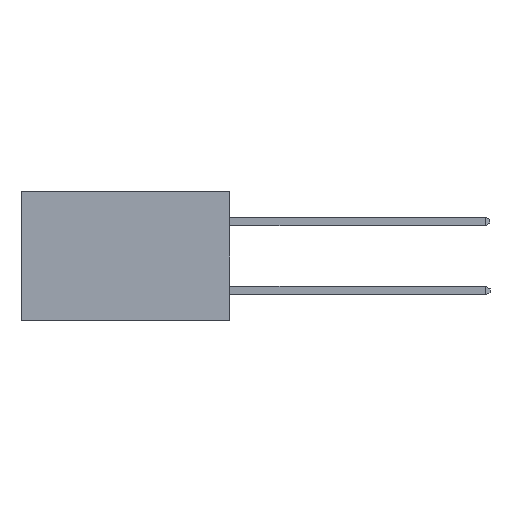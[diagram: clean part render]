
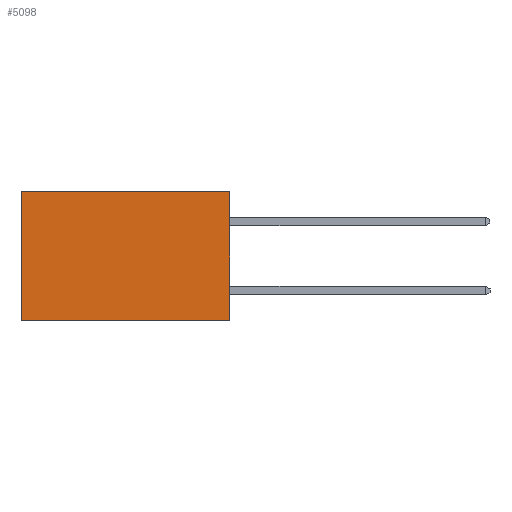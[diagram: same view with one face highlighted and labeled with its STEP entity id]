
A CAD part, left-side view. The second image highlights one B-rep face of the part: STEP entity #5098.
In plain terms, the highlighted planar face has unit normal (-1, 0, 0).
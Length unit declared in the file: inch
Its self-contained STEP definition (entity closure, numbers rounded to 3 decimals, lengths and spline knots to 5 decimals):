
#78 = LINE ( 'NONE', #9357, #5470 ) ;
#97 = LINE ( 'NONE', #1122, #5834 ) ;
#452 = LINE ( 'NONE', #4687, #1757 ) ;
#586 = CARTESIAN_POINT ( 'NONE',  ( 0.2615, 0.6, 0. ) ) ;
#973 = EDGE_CURVE ( 'NONE', #6208, #2812, #78, .T. ) ;
#1024 = CARTESIAN_POINT ( 'NONE',  ( 0.2615, 0.6, -0.37 ) ) ;
#1122 = CARTESIAN_POINT ( 'NONE',  ( 0.2615, 0., 0. ) ) ;
#1213 = CARTESIAN_POINT ( 'NONE',  ( 0.2615, 0.6, -0.37 ) ) ;
#1757 = VECTOR ( 'NONE', #4722, 39.37008 ) ;
#2053 = EDGE_CURVE ( 'NONE', #6208, #2196, #97, .T. ) ;
#2196 = VERTEX_POINT ( 'NONE', #586 ) ;
#2489 = CARTESIAN_POINT ( 'NONE',  ( 0.2615, 0., -0.37 ) ) ;
#2812 = VERTEX_POINT ( 'NONE', #5311 ) ;
#3044 = LINE ( 'NONE', #1213, #5937 ) ;
#3311 = ORIENTED_EDGE ( 'NONE', *, *, #7819, .T. ) ;
#3485 = DIRECTION ( 'NONE',  ( 0., 0., -1. ) ) ;
#3558 = FACE_OUTER_BOUND ( 'NONE', #4584, .T. ) ;
#3773 = ORIENTED_EDGE ( 'NONE', *, *, #2053, .T. ) ;
#4584 = EDGE_LOOP ( 'NONE', ( #3311, #8832, #4750, #3773 ) ) ;
#4687 = CARTESIAN_POINT ( 'NONE',  ( 0.2615, 0., -0.37 ) ) ;
#4722 = DIRECTION ( 'NONE',  ( 0., 1., 0. ) ) ;
#4749 = CARTESIAN_POINT ( 'NONE',  ( 0.2615, 0., 0. ) ) ;
#4750 = ORIENTED_EDGE ( 'NONE', *, *, #973, .F. ) ;
#5015 = DIRECTION ( 'NONE',  ( 0., 0., -1. ) ) ;
#5098 = ADVANCED_FACE ( 'NONE', ( #3558 ), #6985, .F. ) ;
#5311 = CARTESIAN_POINT ( 'NONE',  ( 0.2615, 0., -0.37 ) ) ;
#5470 = VECTOR ( 'NONE', #3485, 39.37008 ) ;
#5568 = DIRECTION ( 'NONE',  ( 1., 0., 0. ) ) ;
#5834 = VECTOR ( 'NONE', #9251, 39.37008 ) ;
#5937 = VECTOR ( 'NONE', #5015, 39.37008 ) ;
#6208 = VERTEX_POINT ( 'NONE', #4749 ) ;
#6985 = PLANE ( 'NONE',  #8529 ) ;
#7781 = DIRECTION ( 'NONE',  ( 0., 0., -1. ) ) ;
#7819 = EDGE_CURVE ( 'NONE', #2196, #8099, #3044, .T. ) ;
#8099 = VERTEX_POINT ( 'NONE', #1024 ) ;
#8529 = AXIS2_PLACEMENT_3D ( 'NONE', #2489, #5568, #7781 ) ;
#8832 = ORIENTED_EDGE ( 'NONE', *, *, #9459, .F. ) ;
#9251 = DIRECTION ( 'NONE',  ( 0., 1., 0. ) ) ;
#9357 = CARTESIAN_POINT ( 'NONE',  ( 0.2615, 0., -0.37 ) ) ;
#9459 = EDGE_CURVE ( 'NONE', #2812, #8099, #452, .T. ) ;
